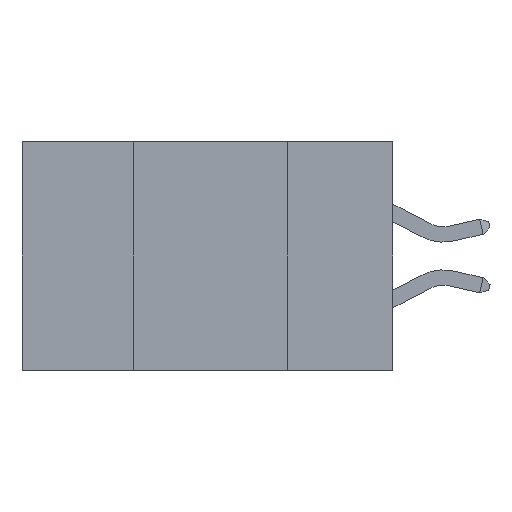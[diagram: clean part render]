
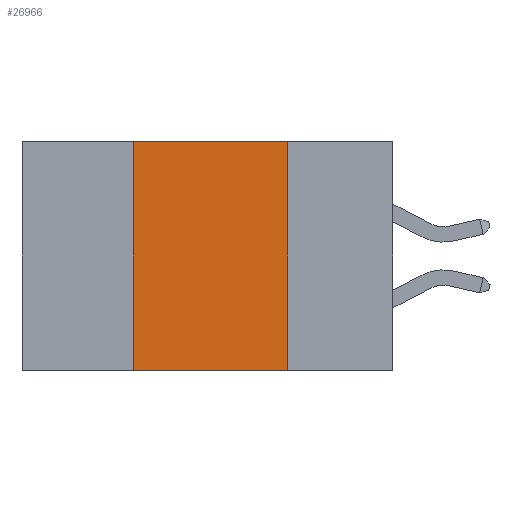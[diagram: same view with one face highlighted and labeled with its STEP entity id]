
A CAD part, left-side view. The second image highlights one B-rep face of the part: STEP entity #26966.
In plain terms, the highlighted planar face has unit normal (-1, 0, 0).
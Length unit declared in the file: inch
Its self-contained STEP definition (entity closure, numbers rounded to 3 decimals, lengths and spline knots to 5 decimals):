
#581 = CARTESIAN_POINT ( 'NONE',  ( 0., 0.17, 0. ) ) ;
#630 = VECTOR ( 'NONE', #36324, 39.37008 ) ;
#2687 = VERTEX_POINT ( 'NONE', #30351 ) ;
#5347 = FACE_OUTER_BOUND ( 'NONE', #37975, .T. ) ;
#5642 = EDGE_CURVE ( 'NONE', #2687, #20988, #19106, .T. ) ;
#5664 = VECTOR ( 'NONE', #32841, 39.37008 ) ;
#6119 = CARTESIAN_POINT ( 'NONE',  ( 0., 0.17, -0.37 ) ) ;
#7434 = ORIENTED_EDGE ( 'NONE', *, *, #5642, .T. ) ;
#8237 = CARTESIAN_POINT ( 'NONE',  ( 0., 0.6, 0. ) ) ;
#9362 = VERTEX_POINT ( 'NONE', #34143 ) ;
#9573 = VERTEX_POINT ( 'NONE', #581 ) ;
#18328 = CARTESIAN_POINT ( 'NONE',  ( 0., 0.42, 0. ) ) ;
#19094 = ORIENTED_EDGE ( 'NONE', *, *, #22538, .F. ) ;
#19106 = LINE ( 'NONE', #36016, #32118 ) ;
#20136 = DIRECTION ( 'NONE',  ( 0., 0., -1. ) ) ;
#20988 = VERTEX_POINT ( 'NONE', #6119 ) ;
#22217 = EDGE_CURVE ( 'NONE', #2687, #9362, #28059, .T. ) ;
#22538 = EDGE_CURVE ( 'NONE', #9573, #20988, #28399, .T. ) ;
#22838 = AXIS2_PLACEMENT_3D ( 'NONE', #8237, #31951, #20136 ) ;
#25116 = CARTESIAN_POINT ( 'NONE',  ( 0., 0.17, 0. ) ) ;
#25752 = LINE ( 'NONE', #30236, #630 ) ;
#26222 = VECTOR ( 'NONE', #33873, 39.37008 ) ;
#26966 = ADVANCED_FACE ( 'NONE', ( #5347 ), #37667, .F. ) ;
#26992 = ORIENTED_EDGE ( 'NONE', *, *, #22217, .F. ) ;
#28059 = LINE ( 'NONE', #18328, #26222 ) ;
#28399 = LINE ( 'NONE', #25116, #5664 ) ;
#30236 = CARTESIAN_POINT ( 'NONE',  ( 0., 0.6, 0. ) ) ;
#30351 = CARTESIAN_POINT ( 'NONE',  ( 0., 0.42, -0.37 ) ) ;
#31951 = DIRECTION ( 'NONE',  ( 1., 0., 0. ) ) ;
#32118 = VECTOR ( 'NONE', #36292, 39.37008 ) ;
#32841 = DIRECTION ( 'NONE',  ( 0., 0., -1. ) ) ;
#33442 = ORIENTED_EDGE ( 'NONE', *, *, #38272, .F. ) ;
#33873 = DIRECTION ( 'NONE',  ( 0., 0., 1. ) ) ;
#34143 = CARTESIAN_POINT ( 'NONE',  ( 0., 0.42, 0. ) ) ;
#36016 = CARTESIAN_POINT ( 'NONE',  ( 0., 0.6, -0.37 ) ) ;
#36292 = DIRECTION ( 'NONE',  ( 0., -1., 0. ) ) ;
#36324 = DIRECTION ( 'NONE',  ( 0., -1., 0. ) ) ;
#37667 = PLANE ( 'NONE',  #22838 ) ;
#37975 = EDGE_LOOP ( 'NONE', ( #19094, #33442, #26992, #7434 ) ) ;
#38272 = EDGE_CURVE ( 'NONE', #9362, #9573, #25752, .T. ) ;
